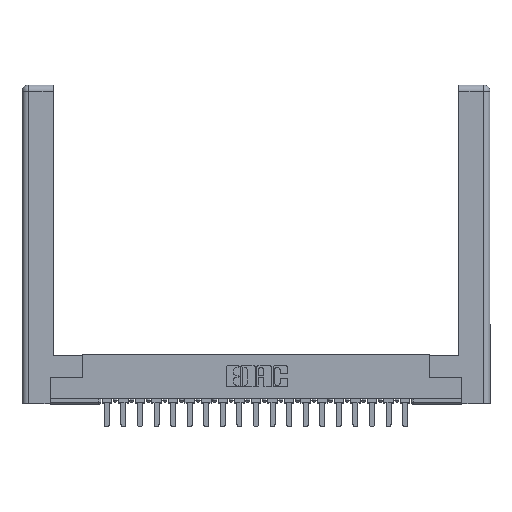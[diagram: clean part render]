
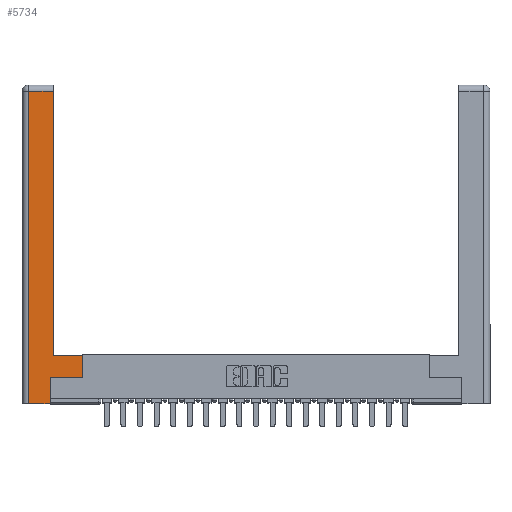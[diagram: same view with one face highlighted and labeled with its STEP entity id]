
A CAD part, top view. The second image highlights one B-rep face of the part: STEP entity #5734.
In plain terms, the highlighted planar face has unit normal (0, 0, 1).
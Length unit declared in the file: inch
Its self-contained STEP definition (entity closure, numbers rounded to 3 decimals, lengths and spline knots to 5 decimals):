
#194 = VECTOR ( 'NONE', #21903, 39.37008 ) ;
#485 = AXIS2_PLACEMENT_3D ( 'NONE', #22170, #1252, #6633 ) ;
#736 = DIRECTION ( 'NONE',  ( 0., 1., 0. ) ) ;
#819 = DIRECTION ( 'NONE',  ( -1., 0., 0. ) ) ;
#1120 = CARTESIAN_POINT ( 'NONE',  ( 0.295, 0.45, 0. ) ) ;
#1252 = DIRECTION ( 'NONE',  ( 0., 0., -1. ) ) ;
#1257 = FACE_OUTER_BOUND ( 'NONE', #3186, .T. ) ;
#1317 = CARTESIAN_POINT ( 'NONE',  ( 0.295, 3., 0. ) ) ;
#2427 = VECTOR ( 'NONE', #6144, 39.37008 ) ;
#2754 = CARTESIAN_POINT ( 'NONE',  ( 0.265, 0., 0. ) ) ;
#2814 = EDGE_CURVE ( 'NONE', #21941, #6091, #2972, .T. ) ;
#2873 = CARTESIAN_POINT ( 'NONE',  ( 0.565, 0.45, 0. ) ) ;
#2972 = LINE ( 'NONE', #1120, #20084 ) ;
#3186 = EDGE_LOOP ( 'NONE', ( #6842, #12424, #21602, #15734, #18273, #13597, #12919, #15416 ) ) ;
#3301 = VECTOR ( 'NONE', #18894, 39.37008 ) ;
#3931 = LINE ( 'NONE', #7893, #18592 ) ;
#4457 = EDGE_CURVE ( 'NONE', #19169, #20449, #13245, .T. ) ;
#5283 = VECTOR ( 'NONE', #7922, 39.37008 ) ;
#5734 = ADVANCED_FACE ( 'NONE', ( #1257 ), #17014, .F. ) ;
#6091 = VERTEX_POINT ( 'NONE', #21627 ) ;
#6140 = CARTESIAN_POINT ( 'NONE',  ( 0.0615, 2.94, 0. ) ) ;
#6144 = DIRECTION ( 'NONE',  ( -1., 0., 0. ) ) ;
#6633 = DIRECTION ( 'NONE',  ( -1., 0., 0. ) ) ;
#6791 = VERTEX_POINT ( 'NONE', #6140 ) ;
#6842 = ORIENTED_EDGE ( 'NONE', *, *, #21009, .T. ) ;
#6930 = CARTESIAN_POINT ( 'NONE',  ( 0.565, 0.245, 0. ) ) ;
#7505 = EDGE_CURVE ( 'NONE', #6791, #21678, #11789, .T. ) ;
#7893 = CARTESIAN_POINT ( 'NONE',  ( 0.265, 0.245, 0. ) ) ;
#7922 = DIRECTION ( 'NONE',  ( 0., -1., 0. ) ) ;
#9293 = VERTEX_POINT ( 'NONE', #2754 ) ;
#10161 = CARTESIAN_POINT ( 'NONE',  ( 0.265, 0., 0. ) ) ;
#10522 = LINE ( 'NONE', #2873, #194 ) ;
#11690 = VERTEX_POINT ( 'NONE', #21824 ) ;
#11789 = LINE ( 'NONE', #12973, #5283 ) ;
#11805 = EDGE_CURVE ( 'NONE', #20449, #21941, #10522, .T. ) ;
#12165 = CARTESIAN_POINT ( 'NONE',  ( 0.565, 0.45, 0. ) ) ;
#12222 = VECTOR ( 'NONE', #15208, 39.37008 ) ;
#12424 = ORIENTED_EDGE ( 'NONE', *, *, #18010, .T. ) ;
#12919 = ORIENTED_EDGE ( 'NONE', *, *, #11805, .T. ) ;
#12973 = CARTESIAN_POINT ( 'NONE',  ( 0.0615, 0., 0. ) ) ;
#13245 = LINE ( 'NONE', #6930, #16761 ) ;
#13293 = CARTESIAN_POINT ( 'NONE',  ( 0.265, 0.245, 0. ) ) ;
#13382 = CARTESIAN_POINT ( 'NONE',  ( 0.0615, 0., 0. ) ) ;
#13597 = ORIENTED_EDGE ( 'NONE', *, *, #4457, .T. ) ;
#14625 = EDGE_CURVE ( 'NONE', #9293, #19169, #3931, .T. ) ;
#15208 = DIRECTION ( 'NONE',  ( 0., 1., 0. ) ) ;
#15416 = ORIENTED_EDGE ( 'NONE', *, *, #2814, .T. ) ;
#15734 = ORIENTED_EDGE ( 'NONE', *, *, #16341, .T. ) ;
#16054 = LINE ( 'NONE', #10161, #3301 ) ;
#16269 = LINE ( 'NONE', #1317, #12222 ) ;
#16341 = EDGE_CURVE ( 'NONE', #21678, #9293, #16054, .T. ) ;
#16761 = VECTOR ( 'NONE', #20809, 39.37008 ) ;
#17014 = PLANE ( 'NONE',  #485 ) ;
#18010 = EDGE_CURVE ( 'NONE', #11690, #6791, #20905, .T. ) ;
#18273 = ORIENTED_EDGE ( 'NONE', *, *, #14625, .T. ) ;
#18592 = VECTOR ( 'NONE', #736, 39.37008 ) ;
#18894 = DIRECTION ( 'NONE',  ( 1., 0., 0. ) ) ;
#19169 = VERTEX_POINT ( 'NONE', #13293 ) ;
#20084 = VECTOR ( 'NONE', #819, 39.37008 ) ;
#20120 = CARTESIAN_POINT ( 'NONE',  ( 0.0615, 2.94, 0. ) ) ;
#20449 = VERTEX_POINT ( 'NONE', #22174 ) ;
#20809 = DIRECTION ( 'NONE',  ( 1., 0., 0. ) ) ;
#20905 = LINE ( 'NONE', #20120, #2427 ) ;
#21009 = EDGE_CURVE ( 'NONE', #6091, #11690, #16269, .T. ) ;
#21602 = ORIENTED_EDGE ( 'NONE', *, *, #7505, .T. ) ;
#21627 = CARTESIAN_POINT ( 'NONE',  ( 0.295, 0.45, 0. ) ) ;
#21678 = VERTEX_POINT ( 'NONE', #13382 ) ;
#21824 = CARTESIAN_POINT ( 'NONE',  ( 0.295, 2.94, 0. ) ) ;
#21903 = DIRECTION ( 'NONE',  ( 0., 1., 0. ) ) ;
#21941 = VERTEX_POINT ( 'NONE', #12165 ) ;
#22170 = CARTESIAN_POINT ( 'NONE',  ( 0., 0., 0. ) ) ;
#22174 = CARTESIAN_POINT ( 'NONE',  ( 0.565, 0.245, 0. ) ) ;
